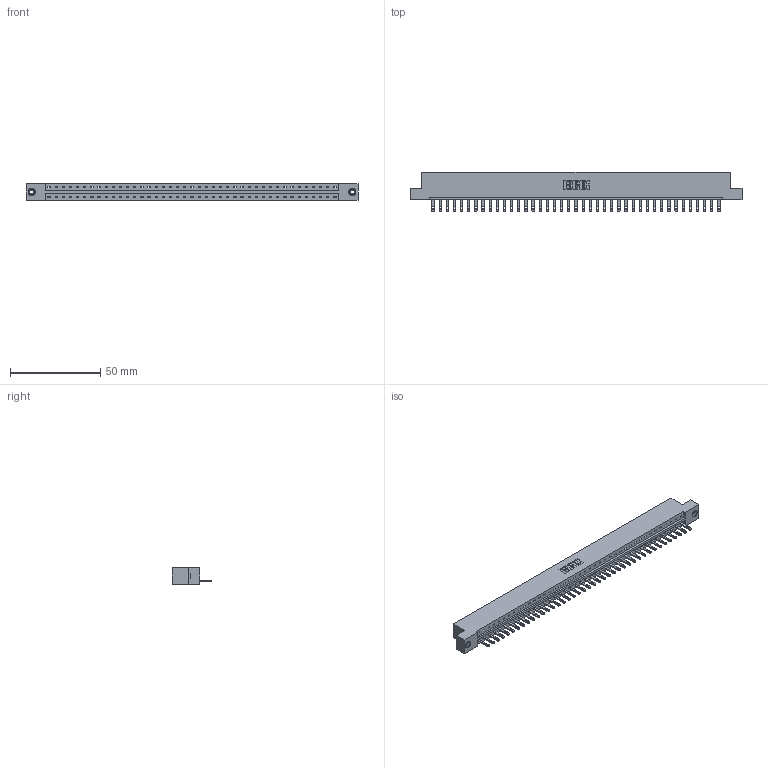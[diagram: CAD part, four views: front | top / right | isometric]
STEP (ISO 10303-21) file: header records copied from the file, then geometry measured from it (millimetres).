
FILE_DESCRIPTION (( 'STEP AP203' ), '1' );
FILE_NAME ('333-041-500-108.STEP', '2018-08-03T15:03:56', ( '' ), ( '' ), 'SwSTEP 2.0', 'SolidWorks 2016', '' );
FILE_SCHEMA (( 'CONFIG_CONTROL_DESIGN' ));
Length unit declared in the file: inch
Products named in the file (4): 345-292-001_345-293-100; 345-250-001_345-250-003-102; 333-041-500-108; 333 Part_Flush - .156 Dia - TI
Assembly tree (44 placements, depth 2):
  333-041-500-108
    333 Part_Flush - .156 Dia - TI
    345-292-001_345-293-100  x41
    345-250-001_345-250-003-102  x2
Bounding box: 184 x 21.85 x 9.4 mm (x, y, z)
Volume: 18525.6 mm3; surface area: 20163.3 mm2
Topology: 44 solids, 44 shells, 2388 faces, 7335 edges, 4882 vertices
Faces by surface type: plane 1578, cylinder 794, cone 12, torus 4
Entity records: 26310 total; most frequent: CARTESIAN_POINT 4520, ORIENTED_EDGE 4490, DIRECTION 3849, EDGE_CURVE 2245, VECTOR 2093, LINE 2093, VERTEX_POINT 1492, AXIS2_PLACEMENT_3D 878
